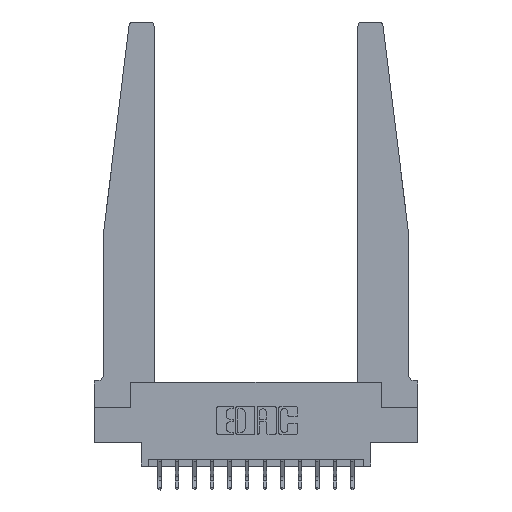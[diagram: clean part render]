
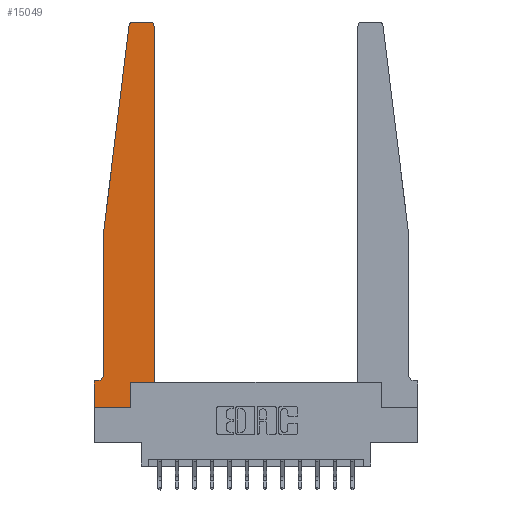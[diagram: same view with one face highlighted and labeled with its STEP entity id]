
A CAD part, top view. The second image highlights one B-rep face of the part: STEP entity #15049.
In plain terms, the highlighted planar face has unit normal (0, 0, 1).
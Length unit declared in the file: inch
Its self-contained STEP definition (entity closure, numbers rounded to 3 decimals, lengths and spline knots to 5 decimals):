
#139 = DIRECTION ( 'NONE',  ( 0., -1., 0. ) ) ;
#149 = ORIENTED_EDGE ( 'NONE', *, *, #1507, .T. ) ;
#412 = CARTESIAN_POINT ( 'NONE',  ( 0.2605, 0.18, 0.37 ) ) ;
#717 = CARTESIAN_POINT ( 'NONE',  ( 0.2605, 0., 0.37 ) ) ;
#1053 = DIRECTION ( 'NONE',  ( 0., 1., 0. ) ) ;
#1140 = VERTEX_POINT ( 'NONE', #16916 ) ;
#1210 = VERTEX_POINT ( 'NONE', #13569 ) ;
#1341 = ORIENTED_EDGE ( 'NONE', *, *, #3735, .T. ) ;
#1452 = CARTESIAN_POINT ( 'NONE',  ( 0.065, 1.25, 0.37 ) ) ;
#1507 = EDGE_CURVE ( 'NONE', #11294, #11790, #14492, .T. ) ;
#1982 = FACE_OUTER_BOUND ( 'NONE', #15322, .T. ) ;
#2286 = EDGE_CURVE ( 'NONE', #10637, #14017, #13854, .T. ) ;
#2400 = AXIS2_PLACEMENT_3D ( 'NONE', #7386, #16576, #8712 ) ;
#2506 = CARTESIAN_POINT ( 'NONE',  ( 0., 0., 0.37 ) ) ;
#2627 = LINE ( 'NONE', #6316, #5284 ) ;
#2791 = VECTOR ( 'NONE', #11671, 39.37008 ) ;
#2986 = CARTESIAN_POINT ( 'NONE',  ( 0.395, 2.75, 0.37 ) ) ;
#3590 = EDGE_CURVE ( 'NONE', #1210, #9008, #9505, .T. ) ;
#3735 = EDGE_CURVE ( 'NONE', #9123, #11294, #14427, .T. ) ;
#4031 = VERTEX_POINT ( 'NONE', #11546 ) ;
#4117 = CIRCLE ( 'NONE', #13216, 0.03 ) ;
#4176 = CARTESIAN_POINT ( 'NONE',  ( 0.25, 2.75, 0.37 ) ) ;
#4221 = CARTESIAN_POINT ( 'NONE',  ( 0.065, 1.25, 0.37 ) ) ;
#4457 = EDGE_CURVE ( 'NONE', #4031, #13552, #4117, .T. ) ;
#4580 = CARTESIAN_POINT ( 'NONE',  ( 0.27653, 2.72, 0.37 ) ) ;
#4767 = ORIENTED_EDGE ( 'NONE', *, *, #4457, .T. ) ;
#4933 = ORIENTED_EDGE ( 'NONE', *, *, #2286, .T. ) ;
#5284 = VECTOR ( 'NONE', #16833, 39.37008 ) ;
#5303 = ORIENTED_EDGE ( 'NONE', *, *, #6835, .T. ) ;
#5753 = CARTESIAN_POINT ( 'NONE',  ( 0., 0.1875, 0.37 ) ) ;
#5812 = CARTESIAN_POINT ( 'NONE',  ( 0., 0.1875, 0.37 ) ) ;
#5841 = AXIS2_PLACEMENT_3D ( 'NONE', #14293, #6427, #15614 ) ;
#5895 = DIRECTION ( 'NONE',  ( 1., 0., 0. ) ) ;
#6077 = ORIENTED_EDGE ( 'NONE', *, *, #7645, .T. ) ;
#6152 = EDGE_CURVE ( 'NONE', #1140, #15025, #8826, .T. ) ;
#6282 = CARTESIAN_POINT ( 'NONE',  ( 0.425, 0.18, 0.37 ) ) ;
#6316 = CARTESIAN_POINT ( 'NONE',  ( 0.2605, 0.18, 0.37 ) ) ;
#6339 = ORIENTED_EDGE ( 'NONE', *, *, #9429, .T. ) ;
#6427 = DIRECTION ( 'NONE',  ( 0., 0., 1. ) ) ;
#6835 = EDGE_CURVE ( 'NONE', #7926, #4031, #12909, .T. ) ;
#7140 = DIRECTION ( 'NONE',  ( 1., 0., 0. ) ) ;
#7288 = CARTESIAN_POINT ( 'NONE',  ( 0., 0., 0.37 ) ) ;
#7386 = CARTESIAN_POINT ( 'NONE',  ( 0.015, 0.2375, 0.37 ) ) ;
#7429 = VECTOR ( 'NONE', #13452, 39.37008 ) ;
#7490 = VECTOR ( 'NONE', #1053, 39.37008 ) ;
#7645 = EDGE_CURVE ( 'NONE', #14017, #9123, #2627, .T. ) ;
#7926 = VERTEX_POINT ( 'NONE', #2986 ) ;
#8712 = DIRECTION ( 'NONE',  ( -1., 0., 0. ) ) ;
#8779 = LINE ( 'NONE', #4221, #15344 ) ;
#8814 = EDGE_CURVE ( 'NONE', #15025, #10637, #16356, .T. ) ;
#8826 = LINE ( 'NONE', #9100, #15387 ) ;
#8970 = CARTESIAN_POINT ( 'NONE',  ( 0.24675, 2.72367, 0.37 ) ) ;
#9008 = VERTEX_POINT ( 'NONE', #10740 ) ;
#9100 = CARTESIAN_POINT ( 'NONE',  ( 0.065, 0.1875, 0.37 ) ) ;
#9123 = VERTEX_POINT ( 'NONE', #412 ) ;
#9429 = EDGE_CURVE ( 'NONE', #11790, #7926, #14269, .T. ) ;
#9445 = DIRECTION ( 'NONE',  ( -0.122, -0.992, 0. ) ) ;
#9505 = LINE ( 'NONE', #1452, #16074 ) ;
#9608 = CARTESIAN_POINT ( 'NONE',  ( 0.425, 0.18, 0.37 ) ) ;
#9821 = CIRCLE ( 'NONE', #2400, 0.05 ) ;
#9859 = ORIENTED_EDGE ( 'NONE', *, *, #14367, .T. ) ;
#10637 = VERTEX_POINT ( 'NONE', #7288 ) ;
#10740 = CARTESIAN_POINT ( 'NONE',  ( 0.065, 0.2375, 0.37 ) ) ;
#10976 = CARTESIAN_POINT ( 'NONE',  ( 0.425, 2.72, 0.37 ) ) ;
#11187 = VECTOR ( 'NONE', #14126, 39.37008 ) ;
#11294 = VERTEX_POINT ( 'NONE', #15289 ) ;
#11541 = CARTESIAN_POINT ( 'NONE',  ( 0., 0., 0.37 ) ) ;
#11546 = CARTESIAN_POINT ( 'NONE',  ( 0.27653, 2.75, 0.37 ) ) ;
#11671 = DIRECTION ( 'NONE',  ( 0., -1., 0. ) ) ;
#11790 = VERTEX_POINT ( 'NONE', #10976 ) ;
#11967 = AXIS2_PLACEMENT_3D ( 'NONE', #5812, #14999, #7140 ) ;
#12048 = DIRECTION ( 'NONE',  ( -1., 0., 0. ) ) ;
#12625 = ORIENTED_EDGE ( 'NONE', *, *, #14044, .T. ) ;
#12771 = ORIENTED_EDGE ( 'NONE', *, *, #3590, .T. ) ;
#12909 = LINE ( 'NONE', #4176, #16822 ) ;
#13216 = AXIS2_PLACEMENT_3D ( 'NONE', #4580, #13776, #5895 ) ;
#13452 = DIRECTION ( 'NONE',  ( 1., 0., 0. ) ) ;
#13552 = VERTEX_POINT ( 'NONE', #8970 ) ;
#13569 = CARTESIAN_POINT ( 'NONE',  ( 0.065, 1.25, 0.37 ) ) ;
#13776 = DIRECTION ( 'NONE',  ( 0., 0., 1. ) ) ;
#13854 = LINE ( 'NONE', #11541, #11187 ) ;
#14017 = VERTEX_POINT ( 'NONE', #717 ) ;
#14044 = EDGE_CURVE ( 'NONE', #9008, #1140, #9821, .T. ) ;
#14126 = DIRECTION ( 'NONE',  ( 1., 0., 0. ) ) ;
#14269 = CIRCLE ( 'NONE', #5841, 0.03 ) ;
#14293 = CARTESIAN_POINT ( 'NONE',  ( 0.395, 2.72, 0.37 ) ) ;
#14367 = EDGE_CURVE ( 'NONE', #13552, #1210, #8779, .T. ) ;
#14427 = LINE ( 'NONE', #9608, #7429 ) ;
#14492 = LINE ( 'NONE', #6282, #7490 ) ;
#14947 = PLANE ( 'NONE',  #11967 ) ;
#14999 = DIRECTION ( 'NONE',  ( 0., 0., 1. ) ) ;
#15025 = VERTEX_POINT ( 'NONE', #5753 ) ;
#15049 = ADVANCED_FACE ( 'NONE', ( #1982 ), #14947, .T. ) ;
#15289 = CARTESIAN_POINT ( 'NONE',  ( 0.425, 0.18, 0.37 ) ) ;
#15322 = EDGE_LOOP ( 'NONE', ( #5303, #4767, #9859, #12771, #12625, #16133, #16080, #4933, #6077, #1341, #149, #6339 ) ) ;
#15344 = VECTOR ( 'NONE', #9445, 39.37008 ) ;
#15387 = VECTOR ( 'NONE', #16963, 39.37008 ) ;
#15614 = DIRECTION ( 'NONE',  ( 1., 0., 0. ) ) ;
#16074 = VECTOR ( 'NONE', #139, 39.37008 ) ;
#16080 = ORIENTED_EDGE ( 'NONE', *, *, #8814, .T. ) ;
#16133 = ORIENTED_EDGE ( 'NONE', *, *, #6152, .T. ) ;
#16356 = LINE ( 'NONE', #2506, #2791 ) ;
#16576 = DIRECTION ( 'NONE',  ( 0., 0., -1. ) ) ;
#16822 = VECTOR ( 'NONE', #12048, 39.37008 ) ;
#16833 = DIRECTION ( 'NONE',  ( 0., 1., 0. ) ) ;
#16916 = CARTESIAN_POINT ( 'NONE',  ( 0.015, 0.1875, 0.37 ) ) ;
#16963 = DIRECTION ( 'NONE',  ( -1., 0., 0. ) ) ;
